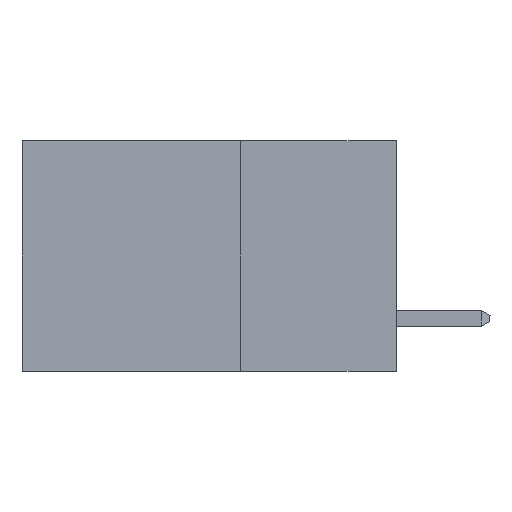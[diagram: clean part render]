
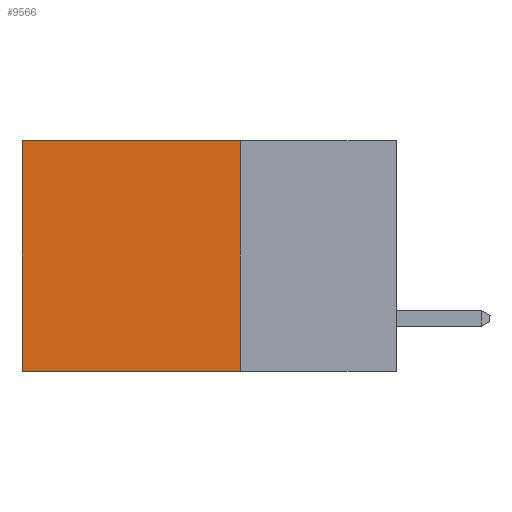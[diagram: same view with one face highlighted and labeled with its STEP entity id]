
A CAD part, left-side view. The second image highlights one B-rep face of the part: STEP entity #9566.
In plain terms, the highlighted planar face has unit normal (-1, 0, 0).
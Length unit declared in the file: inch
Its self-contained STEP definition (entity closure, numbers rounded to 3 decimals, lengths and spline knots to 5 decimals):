
#247 = CARTESIAN_POINT ( 'NONE',  ( 0.298, 0.25, 0. ) ) ;
#299 = VERTEX_POINT ( 'NONE', #10756 ) ;
#874 = EDGE_LOOP ( 'NONE', ( #8345, #2273, #10673, #3316 ) ) ;
#1180 = FACE_OUTER_BOUND ( 'NONE', #874, .T. ) ;
#1596 = VECTOR ( 'NONE', #3356, 39.37008 ) ;
#1760 = CARTESIAN_POINT ( 'NONE',  ( 0.298, 0.25, -0.37 ) ) ;
#1786 = DIRECTION ( 'NONE',  ( 1., 0., 0. ) ) ;
#2073 = EDGE_CURVE ( 'NONE', #3660, #299, #6485, .T. ) ;
#2273 = ORIENTED_EDGE ( 'NONE', *, *, #5402, .F. ) ;
#3316 = ORIENTED_EDGE ( 'NONE', *, *, #4948, .T. ) ;
#3356 = DIRECTION ( 'NONE',  ( 0., 0., -1. ) ) ;
#3613 = LINE ( 'NONE', #7723, #8982 ) ;
#3660 = VERTEX_POINT ( 'NONE', #6290 ) ;
#3723 = DIRECTION ( 'NONE',  ( 0., 1., 0. ) ) ;
#3759 = CARTESIAN_POINT ( 'NONE',  ( 0.298, 0.6, 0. ) ) ;
#4747 = EDGE_CURVE ( 'NONE', #5639, #10473, #8572, .T. ) ;
#4922 = CARTESIAN_POINT ( 'NONE',  ( 0.298, 0.6, -0.37 ) ) ;
#4948 = EDGE_CURVE ( 'NONE', #3660, #5639, #3613, .T. ) ;
#5038 = CARTESIAN_POINT ( 'NONE',  ( 0.298, 0.6, 0. ) ) ;
#5155 = CARTESIAN_POINT ( 'NONE',  ( 0.298, 0.25, 0. ) ) ;
#5243 = PLANE ( 'NONE',  #5690 ) ;
#5402 = EDGE_CURVE ( 'NONE', #299, #10473, #9507, .T. ) ;
#5639 = VERTEX_POINT ( 'NONE', #5038 ) ;
#5690 = AXIS2_PLACEMENT_3D ( 'NONE', #247, #1786, #7823 ) ;
#6290 = CARTESIAN_POINT ( 'NONE',  ( 0.298, 0.25, 0. ) ) ;
#6485 = LINE ( 'NONE', #5155, #1596 ) ;
#7712 = DIRECTION ( 'NONE',  ( 0., 1., 0. ) ) ;
#7723 = CARTESIAN_POINT ( 'NONE',  ( 0.298, 0.25, 0. ) ) ;
#7823 = DIRECTION ( 'NONE',  ( 0., 0., -1. ) ) ;
#8345 = ORIENTED_EDGE ( 'NONE', *, *, #4747, .T. ) ;
#8572 = LINE ( 'NONE', #3759, #10291 ) ;
#8574 = VECTOR ( 'NONE', #7712, 39.37008 ) ;
#8982 = VECTOR ( 'NONE', #3723, 39.37008 ) ;
#9507 = LINE ( 'NONE', #1760, #8574 ) ;
#9566 = ADVANCED_FACE ( 'NONE', ( #1180 ), #5243, .F. ) ;
#10291 = VECTOR ( 'NONE', #10655, 39.37008 ) ;
#10473 = VERTEX_POINT ( 'NONE', #4922 ) ;
#10655 = DIRECTION ( 'NONE',  ( 0., 0., -1. ) ) ;
#10673 = ORIENTED_EDGE ( 'NONE', *, *, #2073, .F. ) ;
#10756 = CARTESIAN_POINT ( 'NONE',  ( 0.298, 0.25, -0.37 ) ) ;
